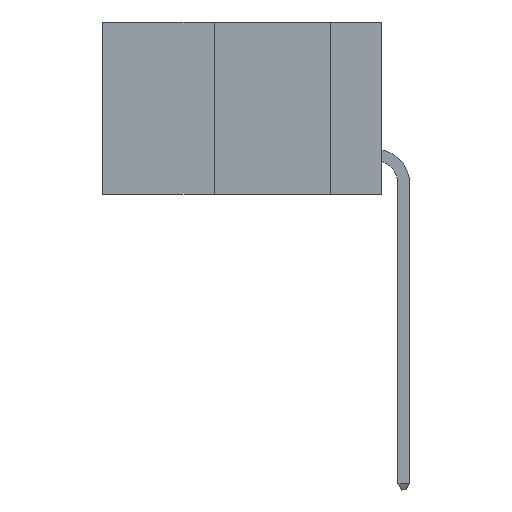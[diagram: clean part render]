
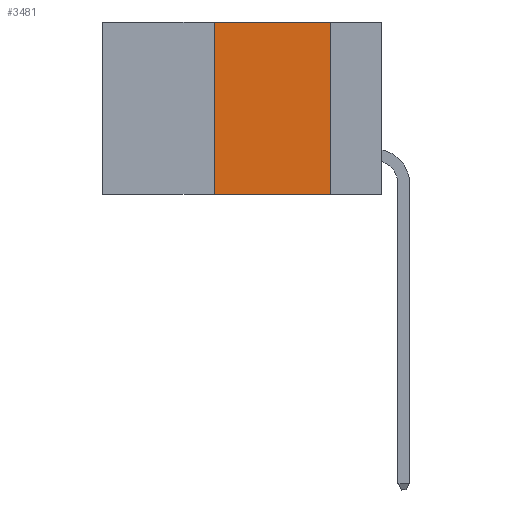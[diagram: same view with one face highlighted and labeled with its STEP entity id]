
A CAD part, left-side view. The second image highlights one B-rep face of the part: STEP entity #3481.
In plain terms, the highlighted planar face has unit normal (-1, 0, 0).
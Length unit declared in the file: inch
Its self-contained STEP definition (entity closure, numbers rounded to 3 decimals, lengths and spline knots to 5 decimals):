
#81 = VERTEX_POINT ( 'NONE', #4668 ) ;
#667 = ORIENTED_EDGE ( 'NONE', *, *, #10183, .F. ) ;
#846 = CARTESIAN_POINT ( 'NONE',  ( 0., 0.36, 0. ) ) ;
#1645 = DIRECTION ( 'NONE',  ( 0., -1., 0. ) ) ;
#1837 = LINE ( 'NONE', #11263, #14437 ) ;
#2258 = PLANE ( 'NONE',  #12731 ) ;
#3118 = DIRECTION ( 'NONE',  ( 0., 0., 1. ) ) ;
#3481 = ADVANCED_FACE ( 'NONE', ( #5038 ), #2258, .F. ) ;
#4462 = LINE ( 'NONE', #846, #9888 ) ;
#4649 = DIRECTION ( 'NONE',  ( 1., 0., 0. ) ) ;
#4668 = CARTESIAN_POINT ( 'NONE',  ( 0., 0.36, -0.37 ) ) ;
#5038 = FACE_OUTER_BOUND ( 'NONE', #12673, .T. ) ;
#5714 = EDGE_CURVE ( 'NONE', #81, #12161, #4462, .T. ) ;
#6034 = CARTESIAN_POINT ( 'NONE',  ( 0., 0.11, -0.37 ) ) ;
#6817 = ORIENTED_EDGE ( 'NONE', *, *, #8081, .F. ) ;
#7205 = DIRECTION ( 'NONE',  ( 0., 0., -1. ) ) ;
#7290 = VECTOR ( 'NONE', #7205, 39.37008 ) ;
#7305 = VERTEX_POINT ( 'NONE', #6034 ) ;
#8081 = EDGE_CURVE ( 'NONE', #9450, #7305, #8562, .T. ) ;
#8426 = CARTESIAN_POINT ( 'NONE',  ( 0., 0.11, 0. ) ) ;
#8562 = LINE ( 'NONE', #8426, #7290 ) ;
#8671 = CARTESIAN_POINT ( 'NONE',  ( 0., 0.6, -0.37 ) ) ;
#9096 = ORIENTED_EDGE ( 'NONE', *, *, #11368, .T. ) ;
#9298 = VECTOR ( 'NONE', #1645, 39.37008 ) ;
#9450 = VERTEX_POINT ( 'NONE', #12170 ) ;
#9888 = VECTOR ( 'NONE', #3118, 39.37008 ) ;
#10134 = DIRECTION ( 'NONE',  ( 0., -1., 0. ) ) ;
#10183 = EDGE_CURVE ( 'NONE', #12161, #9450, #1837, .T. ) ;
#10410 = CARTESIAN_POINT ( 'NONE',  ( 0., 0.6, 0. ) ) ;
#11263 = CARTESIAN_POINT ( 'NONE',  ( 0., 0.6, 0. ) ) ;
#11368 = EDGE_CURVE ( 'NONE', #81, #7305, #13111, .T. ) ;
#12161 = VERTEX_POINT ( 'NONE', #13797 ) ;
#12170 = CARTESIAN_POINT ( 'NONE',  ( 0., 0.11, 0. ) ) ;
#12345 = ORIENTED_EDGE ( 'NONE', *, *, #5714, .F. ) ;
#12673 = EDGE_LOOP ( 'NONE', ( #6817, #667, #12345, #9096 ) ) ;
#12731 = AXIS2_PLACEMENT_3D ( 'NONE', #10410, #4649, #12743 ) ;
#12743 = DIRECTION ( 'NONE',  ( 0., 0., -1. ) ) ;
#13111 = LINE ( 'NONE', #8671, #9298 ) ;
#13797 = CARTESIAN_POINT ( 'NONE',  ( 0., 0.36, 0. ) ) ;
#14437 = VECTOR ( 'NONE', #10134, 39.37008 ) ;
